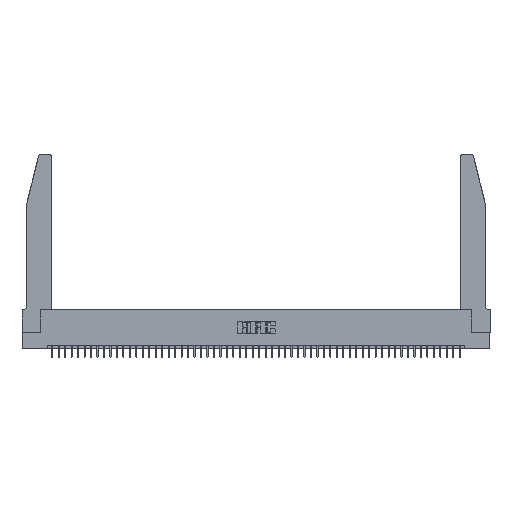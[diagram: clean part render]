
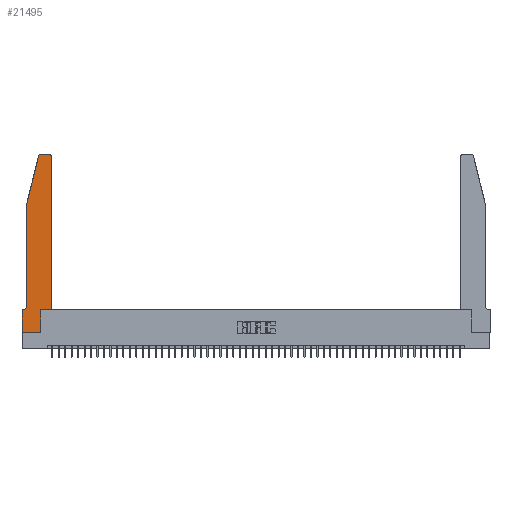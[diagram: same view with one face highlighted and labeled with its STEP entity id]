
A CAD part, top view. The second image highlights one B-rep face of the part: STEP entity #21495.
In plain terms, the highlighted planar face has unit normal (0, 0, 1).
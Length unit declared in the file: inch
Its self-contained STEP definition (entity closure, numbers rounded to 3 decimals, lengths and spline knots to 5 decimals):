
#404 = AXIS2_PLACEMENT_3D ( 'NONE', #30294, #41907, #46369 ) ;
#805 = ORIENTED_EDGE ( 'NONE', *, *, #49285, .T. ) ;
#1568 = CARTESIAN_POINT ( 'NONE',  ( 0.0755, 2., 0.37 ) ) ;
#1836 = VERTEX_POINT ( 'NONE', #31521 ) ;
#2425 = LINE ( 'NONE', #14838, #49091 ) ;
#3309 = DIRECTION ( 'NONE',  ( 0., -1., 0. ) ) ;
#3559 = LINE ( 'NONE', #40219, #37830 ) ;
#4204 = LINE ( 'NONE', #16345, #36911 ) ;
#4636 = VERTEX_POINT ( 'NONE', #44492 ) ;
#5044 = DIRECTION ( 'NONE',  ( -0.239, -0.971, 0. ) ) ;
#5414 = ORIENTED_EDGE ( 'NONE', *, *, #16009, .T. ) ;
#5556 = CIRCLE ( 'NONE', #35040, 0.07 ) ;
#7331 = ORIENTED_EDGE ( 'NONE', *, *, #49086, .T. ) ;
#7682 = CARTESIAN_POINT ( 'NONE',  ( 0.0755, 0.42, 0.37 ) ) ;
#7777 = VERTEX_POINT ( 'NONE', #45009 ) ;
#9156 = VERTEX_POINT ( 'NONE', #36379 ) ;
#9802 = LINE ( 'NONE', #26111, #48868 ) ;
#9822 = CARTESIAN_POINT ( 'NONE',  ( 0., 0.35, 0.37 ) ) ;
#12166 = DIRECTION ( 'NONE',  ( 1., 0., 0. ) ) ;
#14838 = CARTESIAN_POINT ( 'NONE',  ( 0.2865, 0.35, 0.37 ) ) ;
#15608 = CIRCLE ( 'NONE', #404, 0.03 ) ;
#15803 = DIRECTION ( 'NONE',  ( -1., 0., 0. ) ) ;
#16009 = EDGE_CURVE ( 'NONE', #24240, #7777, #40857, .T. ) ;
#16345 = CARTESIAN_POINT ( 'NONE',  ( 0.0755, 0.35, 0.37 ) ) ;
#16422 = CARTESIAN_POINT ( 'NONE',  ( 0.25487, 2.72718, 0.37 ) ) ;
#17186 = LINE ( 'NONE', #33019, #17657 ) ;
#17657 = VECTOR ( 'NONE', #48313, 39.37008 ) ;
#18086 = DIRECTION ( 'NONE',  ( 1., 0., 0. ) ) ;
#18127 = VERTEX_POINT ( 'NONE', #1568 ) ;
#18338 = CARTESIAN_POINT ( 'NONE',  ( 0., 0.35, 0.37 ) ) ;
#18431 = ORIENTED_EDGE ( 'NONE', *, *, #49134, .T. ) ;
#19247 = VERTEX_POINT ( 'NONE', #7682 ) ;
#19284 = EDGE_CURVE ( 'NONE', #7777, #29753, #47928, .T. ) ;
#19762 = CARTESIAN_POINT ( 'NONE',  ( 0.2605, 2.75, 0.37 ) ) ;
#21318 = EDGE_CURVE ( 'NONE', #45735, #1836, #29183, .T. ) ;
#21495 = ADVANCED_FACE ( 'NONE', ( #46307 ), #29963, .T. ) ;
#22345 = VERTEX_POINT ( 'NONE', #41090 ) ;
#22674 = AXIS2_PLACEMENT_3D ( 'NONE', #36692, #49854, #37194 ) ;
#23118 = EDGE_CURVE ( 'NONE', #1836, #50975, #31955, .T. ) ;
#24240 = VERTEX_POINT ( 'NONE', #26479 ) ;
#24547 = ORIENTED_EDGE ( 'NONE', *, *, #40634, .T. ) ;
#25323 = EDGE_LOOP ( 'NONE', ( #5414, #39225, #7331, #24547, #51719, #44880, #37775, #47388, #41984, #805, #18431, #49811 ) ) ;
#25890 = VECTOR ( 'NONE', #15803, 39.37008 ) ;
#26022 = EDGE_CURVE ( 'NONE', #50975, #9156, #2425, .T. ) ;
#26111 = CARTESIAN_POINT ( 'NONE',  ( 0.4505, 0.35, 0.37 ) ) ;
#26148 = DIRECTION ( 'NONE',  ( 0., 1., 0. ) ) ;
#26479 = CARTESIAN_POINT ( 'NONE',  ( 0.4205, 2.75, 0.37 ) ) ;
#27224 = EDGE_CURVE ( 'NONE', #22345, #24240, #15608, .T. ) ;
#28505 = VERTEX_POINT ( 'NONE', #41471 ) ;
#28608 = VECTOR ( 'NONE', #5044, 39.37008 ) ;
#29183 = LINE ( 'NONE', #41064, #37932 ) ;
#29520 = CARTESIAN_POINT ( 'NONE',  ( 0.2865, 0., 0.37 ) ) ;
#29753 = VERTEX_POINT ( 'NONE', #16422 ) ;
#29963 = PLANE ( 'NONE',  #47244 ) ;
#30294 = CARTESIAN_POINT ( 'NONE',  ( 0.4205, 2.72, 0.37 ) ) ;
#31521 = CARTESIAN_POINT ( 'NONE',  ( 0., 0., 0.37 ) ) ;
#31955 = LINE ( 'NONE', #48019, #44831 ) ;
#32238 = CARTESIAN_POINT ( 'NONE',  ( 0.0755, 2., 0.37 ) ) ;
#33019 = CARTESIAN_POINT ( 'NONE',  ( 0.4505, 0.35, 0.37 ) ) ;
#34798 = DIRECTION ( 'NONE',  ( -1., 0., 0. ) ) ;
#35040 = AXIS2_PLACEMENT_3D ( 'NONE', #50627, #51157, #34798 ) ;
#35117 = EDGE_CURVE ( 'NONE', #19247, #28505, #5556, .T. ) ;
#36178 = LINE ( 'NONE', #32238, #28608 ) ;
#36379 = CARTESIAN_POINT ( 'NONE',  ( 0.2865, 0.35, 0.37 ) ) ;
#36692 = CARTESIAN_POINT ( 'NONE',  ( 0.284, 2.72, 0.37 ) ) ;
#36911 = VECTOR ( 'NONE', #51960, 39.37008 ) ;
#37194 = DIRECTION ( 'NONE',  ( 1., 0., 0. ) ) ;
#37775 = ORIENTED_EDGE ( 'NONE', *, *, #21318, .T. ) ;
#37830 = VECTOR ( 'NONE', #3309, 39.37008 ) ;
#37932 = VECTOR ( 'NONE', #48698, 39.37008 ) ;
#39225 = ORIENTED_EDGE ( 'NONE', *, *, #19284, .T. ) ;
#39778 = EDGE_CURVE ( 'NONE', #28505, #45735, #4204, .T. ) ;
#40219 = CARTESIAN_POINT ( 'NONE',  ( 0.0755, 2., 0.37 ) ) ;
#40634 = EDGE_CURVE ( 'NONE', #18127, #19247, #3559, .T. ) ;
#40857 = LINE ( 'NONE', #19762, #25890 ) ;
#41064 = CARTESIAN_POINT ( 'NONE',  ( 0., 0., 0.37 ) ) ;
#41090 = CARTESIAN_POINT ( 'NONE',  ( 0.4505, 2.72, 0.37 ) ) ;
#41471 = CARTESIAN_POINT ( 'NONE',  ( 0.0055, 0.35, 0.37 ) ) ;
#41907 = DIRECTION ( 'NONE',  ( 0., 0., 1. ) ) ;
#41984 = ORIENTED_EDGE ( 'NONE', *, *, #26022, .T. ) ;
#44492 = CARTESIAN_POINT ( 'NONE',  ( 0.4505, 0.35, 0.37 ) ) ;
#44831 = VECTOR ( 'NONE', #12166, 39.37008 ) ;
#44880 = ORIENTED_EDGE ( 'NONE', *, *, #39778, .T. ) ;
#45009 = CARTESIAN_POINT ( 'NONE',  ( 0.284, 2.75, 0.37 ) ) ;
#45735 = VERTEX_POINT ( 'NONE', #9822 ) ;
#46307 = FACE_OUTER_BOUND ( 'NONE', #25323, .T. ) ;
#46369 = DIRECTION ( 'NONE',  ( 1., 0., 0. ) ) ;
#46705 = DIRECTION ( 'NONE',  ( 1., 0., 0. ) ) ;
#47244 = AXIS2_PLACEMENT_3D ( 'NONE', #18338, #50525, #18086 ) ;
#47388 = ORIENTED_EDGE ( 'NONE', *, *, #23118, .T. ) ;
#47928 = CIRCLE ( 'NONE', #22674, 0.03 ) ;
#48019 = CARTESIAN_POINT ( 'NONE',  ( 0., 0., 0.37 ) ) ;
#48313 = DIRECTION ( 'NONE',  ( 0., 1., 0. ) ) ;
#48698 = DIRECTION ( 'NONE',  ( 0., -1., 0. ) ) ;
#48868 = VECTOR ( 'NONE', #46705, 39.37008 ) ;
#49086 = EDGE_CURVE ( 'NONE', #29753, #18127, #36178, .T. ) ;
#49091 = VECTOR ( 'NONE', #26148, 39.37008 ) ;
#49134 = EDGE_CURVE ( 'NONE', #4636, #22345, #17186, .T. ) ;
#49285 = EDGE_CURVE ( 'NONE', #9156, #4636, #9802, .T. ) ;
#49811 = ORIENTED_EDGE ( 'NONE', *, *, #27224, .T. ) ;
#49854 = DIRECTION ( 'NONE',  ( 0., 0., 1. ) ) ;
#50525 = DIRECTION ( 'NONE',  ( 0., 0., 1. ) ) ;
#50627 = CARTESIAN_POINT ( 'NONE',  ( 0.0055, 0.42, 0.37 ) ) ;
#50975 = VERTEX_POINT ( 'NONE', #29520 ) ;
#51157 = DIRECTION ( 'NONE',  ( 0., 0., -1. ) ) ;
#51719 = ORIENTED_EDGE ( 'NONE', *, *, #35117, .T. ) ;
#51960 = DIRECTION ( 'NONE',  ( -1., 0., 0. ) ) ;
